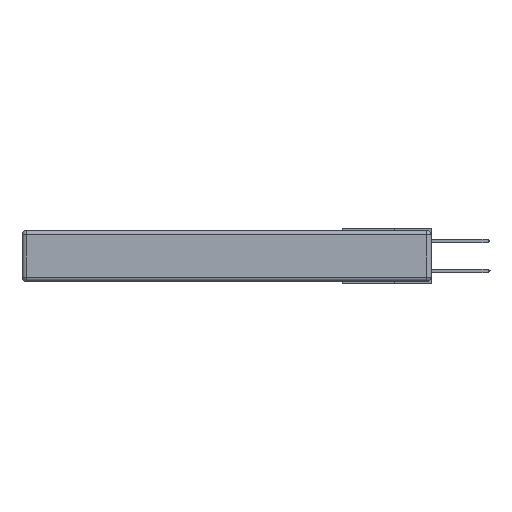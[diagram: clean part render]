
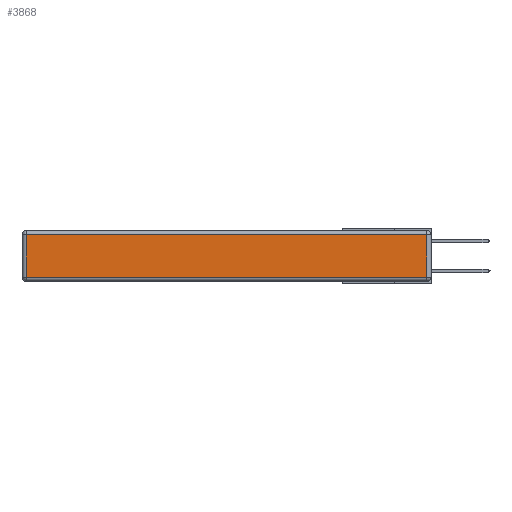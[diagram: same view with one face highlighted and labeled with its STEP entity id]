
A CAD part, left-side view. The second image highlights one B-rep face of the part: STEP entity #3868.
In plain terms, the highlighted planar face has unit normal (-1, 0, 0).
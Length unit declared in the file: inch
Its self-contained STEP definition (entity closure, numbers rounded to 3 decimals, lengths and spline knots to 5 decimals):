
#80 = EDGE_CURVE ( 'NONE', #7126, #4989, #13095, .T. ) ;
#151 = DIRECTION ( 'NONE',  ( 0., 1., 0. ) ) ;
#445 = DIRECTION ( 'NONE',  ( -1., 0., 0. ) ) ;
#744 = VERTEX_POINT ( 'NONE', #8629 ) ;
#1544 = CARTESIAN_POINT ( 'NONE',  ( 0., 0.03, -0.03 ) ) ;
#2425 = CARTESIAN_POINT ( 'NONE',  ( 0., 0.03, -0.313 ) ) ;
#2944 = CARTESIAN_POINT ( 'NONE',  ( 0., 0., -0.343 ) ) ;
#3620 = CARTESIAN_POINT ( 'NONE',  ( 0., 2.72, -0.03 ) ) ;
#3868 = ADVANCED_FACE ( 'NONE', ( #9821 ), #15802, .T. ) ;
#4164 = VECTOR ( 'NONE', #16323, 39.37008 ) ;
#4897 = ORIENTED_EDGE ( 'NONE', *, *, #80, .T. ) ;
#4989 = VERTEX_POINT ( 'NONE', #3620 ) ;
#7126 = VERTEX_POINT ( 'NONE', #1544 ) ;
#8606 = CARTESIAN_POINT ( 'NONE',  ( 0., 0., -0.313 ) ) ;
#8629 = CARTESIAN_POINT ( 'NONE',  ( 0., 2.72, -0.313 ) ) ;
#8978 = CARTESIAN_POINT ( 'NONE',  ( 0., 0.03, -0.343 ) ) ;
#9201 = DIRECTION ( 'NONE',  ( 0., 0., -1. ) ) ;
#9270 = ORIENTED_EDGE ( 'NONE', *, *, #12213, .T. ) ;
#9821 = FACE_OUTER_BOUND ( 'NONE', #13489, .T. ) ;
#9992 = VECTOR ( 'NONE', #9201, 39.37008 ) ;
#10577 = DIRECTION ( 'NONE',  ( 0., 0., 1. ) ) ;
#10790 = LINE ( 'NONE', #8606, #4164 ) ;
#11001 = LINE ( 'NONE', #8978, #14421 ) ;
#11162 = AXIS2_PLACEMENT_3D ( 'NONE', #2944, #445, #10577 ) ;
#11678 = EDGE_CURVE ( 'NONE', #12158, #7126, #11001, .T. ) ;
#11724 = CARTESIAN_POINT ( 'NONE',  ( 0., 2.75, -0.03 ) ) ;
#11879 = EDGE_CURVE ( 'NONE', #4989, #744, #16219, .T. ) ;
#12158 = VERTEX_POINT ( 'NONE', #2425 ) ;
#12213 = EDGE_CURVE ( 'NONE', #744, #12158, #10790, .T. ) ;
#13095 = LINE ( 'NONE', #11724, #16110 ) ;
#13489 = EDGE_LOOP ( 'NONE', ( #9270, #15921, #4897, #14971 ) ) ;
#14289 = CARTESIAN_POINT ( 'NONE',  ( 0., 2.72, -0.343 ) ) ;
#14421 = VECTOR ( 'NONE', #15402, 39.37008 ) ;
#14971 = ORIENTED_EDGE ( 'NONE', *, *, #11879, .T. ) ;
#15402 = DIRECTION ( 'NONE',  ( 0., 0., 1. ) ) ;
#15802 = PLANE ( 'NONE',  #11162 ) ;
#15921 = ORIENTED_EDGE ( 'NONE', *, *, #11678, .T. ) ;
#16110 = VECTOR ( 'NONE', #151, 39.37008 ) ;
#16219 = LINE ( 'NONE', #14289, #9992 ) ;
#16323 = DIRECTION ( 'NONE',  ( 0., -1., 0. ) ) ;
